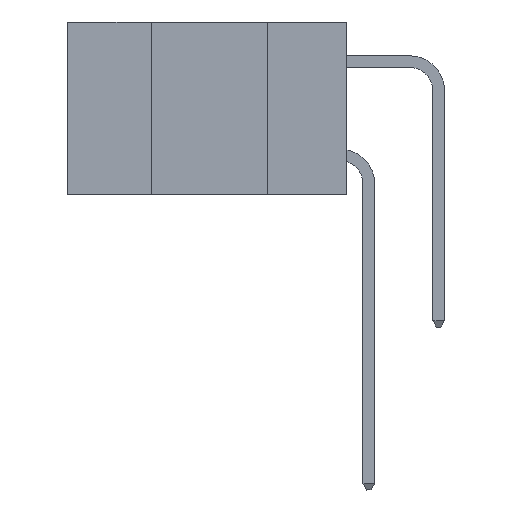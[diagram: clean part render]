
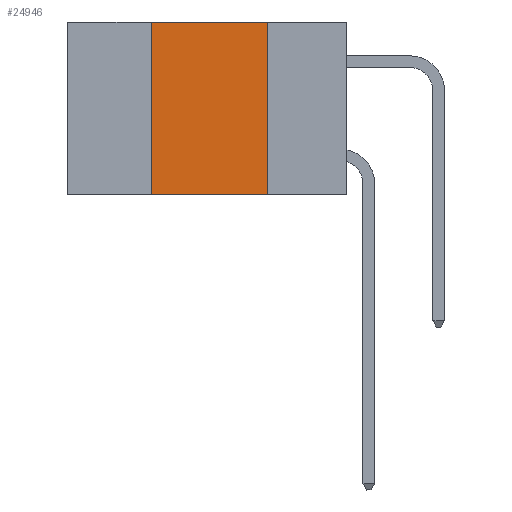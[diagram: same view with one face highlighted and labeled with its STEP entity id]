
A CAD part, left-side view. The second image highlights one B-rep face of the part: STEP entity #24946.
In plain terms, the highlighted planar face has unit normal (-1, 0, 0).
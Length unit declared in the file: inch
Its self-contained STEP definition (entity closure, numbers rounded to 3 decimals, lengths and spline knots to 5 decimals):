
#19 = LINE ( 'NONE', #4249, #21315 ) ;
#2283 = ORIENTED_EDGE ( 'NONE', *, *, #21288, .F. ) ;
#2382 = VERTEX_POINT ( 'NONE', #4638 ) ;
#3077 = CARTESIAN_POINT ( 'NONE',  ( 0., 0.42, 0. ) ) ;
#3933 = DIRECTION ( 'NONE',  ( 0., -1., 0. ) ) ;
#4249 = CARTESIAN_POINT ( 'NONE',  ( 0., 0.6, -0.37 ) ) ;
#4518 = ORIENTED_EDGE ( 'NONE', *, *, #11855, .F. ) ;
#4568 = DIRECTION ( 'NONE',  ( 1., 0., 0. ) ) ;
#4638 = CARTESIAN_POINT ( 'NONE',  ( 0., 0.17, -0.37 ) ) ;
#5709 = EDGE_CURVE ( 'NONE', #21925, #2382, #19, .T. ) ;
#6112 = FACE_OUTER_BOUND ( 'NONE', #9127, .T. ) ;
#8530 = ORIENTED_EDGE ( 'NONE', *, *, #17428, .F. ) ;
#9127 = EDGE_LOOP ( 'NONE', ( #2283, #8530, #4518, #18033 ) ) ;
#9785 = LINE ( 'NONE', #3077, #12277 ) ;
#10074 = CARTESIAN_POINT ( 'NONE',  ( 0., 0.42, -0.37 ) ) ;
#10238 = CARTESIAN_POINT ( 'NONE',  ( 0., 0.42, 0. ) ) ;
#11855 = EDGE_CURVE ( 'NONE', #21925, #22390, #9785, .T. ) ;
#12277 = VECTOR ( 'NONE', #15427, 39.37008 ) ;
#12315 = CARTESIAN_POINT ( 'NONE',  ( 0., 0.17, 0. ) ) ;
#13789 = LINE ( 'NONE', #12315, #21087 ) ;
#15427 = DIRECTION ( 'NONE',  ( 0., 0., 1. ) ) ;
#15742 = VERTEX_POINT ( 'NONE', #25507 ) ;
#15846 = LINE ( 'NONE', #21422, #20491 ) ;
#16344 = CARTESIAN_POINT ( 'NONE',  ( 0., 0.6, 0. ) ) ;
#17428 = EDGE_CURVE ( 'NONE', #22390, #15742, #15846, .T. ) ;
#17972 = DIRECTION ( 'NONE',  ( 0., 0., -1. ) ) ;
#18033 = ORIENTED_EDGE ( 'NONE', *, *, #5709, .T. ) ;
#18351 = DIRECTION ( 'NONE',  ( 0., 0., -1. ) ) ;
#20323 = AXIS2_PLACEMENT_3D ( 'NONE', #16344, #4568, #17972 ) ;
#20491 = VECTOR ( 'NONE', #3933, 39.37008 ) ;
#21087 = VECTOR ( 'NONE', #18351, 39.37008 ) ;
#21288 = EDGE_CURVE ( 'NONE', #15742, #2382, #13789, .T. ) ;
#21315 = VECTOR ( 'NONE', #23624, 39.37008 ) ;
#21422 = CARTESIAN_POINT ( 'NONE',  ( 0., 0.6, 0. ) ) ;
#21925 = VERTEX_POINT ( 'NONE', #10074 ) ;
#22390 = VERTEX_POINT ( 'NONE', #10238 ) ;
#23624 = DIRECTION ( 'NONE',  ( 0., -1., 0. ) ) ;
#24137 = PLANE ( 'NONE',  #20323 ) ;
#24946 = ADVANCED_FACE ( 'NONE', ( #6112 ), #24137, .F. ) ;
#25507 = CARTESIAN_POINT ( 'NONE',  ( 0., 0.17, 0. ) ) ;
